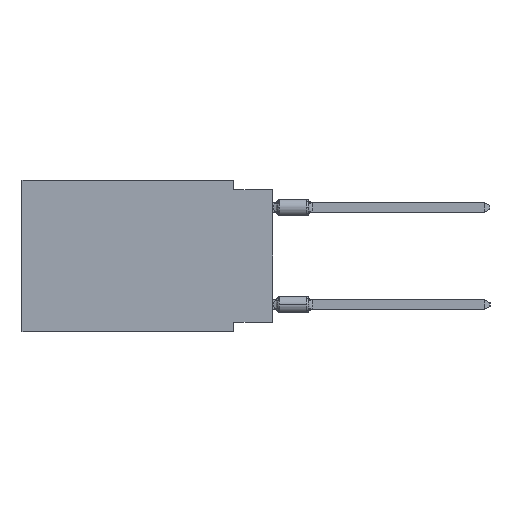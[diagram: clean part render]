
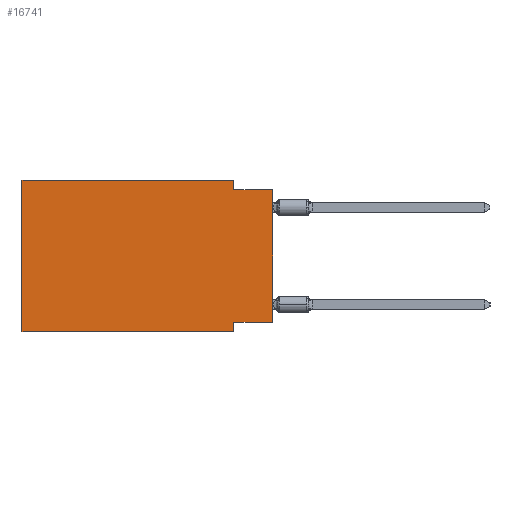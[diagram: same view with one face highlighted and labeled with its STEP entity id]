
A CAD part, left-side view. The second image highlights one B-rep face of the part: STEP entity #16741.
In plain terms, the highlighted planar face has unit normal (-1, 0, 0).
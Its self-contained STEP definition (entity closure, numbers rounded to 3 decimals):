
#205 = ORIENTED_EDGE ( 'NONE', *, *, #2849, .T. ) ;
#939 = EDGE_CURVE ( 'NONE', #19155, #3711, #29981, .T. ) ;
#1609 = CARTESIAN_POINT ( 'NONE',  ( 0., 0., -0.635 ) ) ;
#1792 = LINE ( 'NONE', #2024, #34343 ) ;
#2024 = CARTESIAN_POINT ( 'NONE',  ( 0., 2.54, 0. ) ) ;
#2849 = EDGE_CURVE ( 'NONE', #19155, #4385, #19594, .T. ) ;
#3100 = DIRECTION ( 'NONE',  ( 0., 0., -1. ) ) ;
#3331 = CARTESIAN_POINT ( 'NONE',  ( 0., 2.54, -9.906 ) ) ;
#3711 = VERTEX_POINT ( 'NONE', #45637 ) ;
#3762 = ORIENTED_EDGE ( 'NONE', *, *, #43737, .F. ) ;
#4385 = VERTEX_POINT ( 'NONE', #47497 ) ;
#5010 = LINE ( 'NONE', #1609, #28268 ) ;
#6751 = CARTESIAN_POINT ( 'NONE',  ( 0., 16.383, 0. ) ) ;
#7453 = DIRECTION ( 'NONE',  ( 0., 0., -1. ) ) ;
#8773 = EDGE_CURVE ( 'NONE', #41549, #30461, #1792, .T. ) ;
#8780 = DIRECTION ( 'NONE',  ( 0., -1., 0. ) ) ;
#9137 = VECTOR ( 'NONE', #18567, 1000. ) ;
#10598 = CARTESIAN_POINT ( 'NONE',  ( 0., 2.54, 0. ) ) ;
#13600 = VERTEX_POINT ( 'NONE', #17166 ) ;
#14380 = CARTESIAN_POINT ( 'NONE',  ( 0., 16.383, 0. ) ) ;
#14560 = VECTOR ( 'NONE', #41555, 1000. ) ;
#15902 = VECTOR ( 'NONE', #7453, 1000. ) ;
#15955 = CARTESIAN_POINT ( 'NONE',  ( 0., 0., 0. ) ) ;
#16059 = EDGE_CURVE ( 'NONE', #31178, #13600, #42051, .T. ) ;
#16741 = ADVANCED_FACE ( 'NONE', ( #35404 ), #47547, .F. ) ;
#17166 = CARTESIAN_POINT ( 'NONE',  ( 0., 2.54, -9.906 ) ) ;
#17244 = DIRECTION ( 'NONE',  ( 0., -1., 0. ) ) ;
#17719 = CARTESIAN_POINT ( 'NONE',  ( 0., 16.383, 0. ) ) ;
#17754 = EDGE_CURVE ( 'NONE', #30461, #4385, #5010, .T. ) ;
#18567 = DIRECTION ( 'NONE',  ( 0., 1., 0. ) ) ;
#19155 = VERTEX_POINT ( 'NONE', #35832 ) ;
#19594 = LINE ( 'NONE', #15955, #33290 ) ;
#20043 = DIRECTION ( 'NONE',  ( 0., -1., 0. ) ) ;
#21623 = ORIENTED_EDGE ( 'NONE', *, *, #939, .F. ) ;
#22936 = CARTESIAN_POINT ( 'NONE',  ( 0., 0., -9.271 ) ) ;
#22998 = DIRECTION ( 'NONE',  ( 0., 0., 1. ) ) ;
#23193 = CARTESIAN_POINT ( 'NONE',  ( 0., 2.54, -0.635 ) ) ;
#24993 = EDGE_CURVE ( 'NONE', #46889, #41549, #25009, .T. ) ;
#25009 = LINE ( 'NONE', #17719, #28607 ) ;
#26446 = ORIENTED_EDGE ( 'NONE', *, *, #8773, .F. ) ;
#28111 = EDGE_CURVE ( 'NONE', #3711, #13600, #44375, .T. ) ;
#28268 = VECTOR ( 'NONE', #20043, 1000. ) ;
#28607 = VECTOR ( 'NONE', #17244, 1000. ) ;
#28971 = AXIS2_PLACEMENT_3D ( 'NONE', #6751, #36377, #3100 ) ;
#29757 = CARTESIAN_POINT ( 'NONE',  ( 0., 16.383, -9.906 ) ) ;
#29981 = LINE ( 'NONE', #22936, #9137 ) ;
#30461 = VERTEX_POINT ( 'NONE', #23193 ) ;
#31178 = VERTEX_POINT ( 'NONE', #29757 ) ;
#33290 = VECTOR ( 'NONE', #22998, 1000. ) ;
#34025 = LINE ( 'NONE', #37918, #14560 ) ;
#34343 = VECTOR ( 'NONE', #38711, 1000. ) ;
#35395 = ORIENTED_EDGE ( 'NONE', *, *, #16059, .T. ) ;
#35404 = FACE_OUTER_BOUND ( 'NONE', #43707, .T. ) ;
#35832 = CARTESIAN_POINT ( 'NONE',  ( 0., 0., -9.271 ) ) ;
#36377 = DIRECTION ( 'NONE',  ( 1., 0., 0. ) ) ;
#36874 = ORIENTED_EDGE ( 'NONE', *, *, #17754, .F. ) ;
#37918 = CARTESIAN_POINT ( 'NONE',  ( 0., 16.383, 0. ) ) ;
#38711 = DIRECTION ( 'NONE',  ( 0., 0., -1. ) ) ;
#40564 = VECTOR ( 'NONE', #8780, 1000. ) ;
#41549 = VERTEX_POINT ( 'NONE', #10598 ) ;
#41555 = DIRECTION ( 'NONE',  ( 0., 0., 1. ) ) ;
#42051 = LINE ( 'NONE', #45452, #40564 ) ;
#43707 = EDGE_LOOP ( 'NONE', ( #205, #36874, #26446, #45635, #3762, #35395, #46642, #21623 ) ) ;
#43737 = EDGE_CURVE ( 'NONE', #31178, #46889, #34025, .T. ) ;
#44375 = LINE ( 'NONE', #3331, #15902 ) ;
#45452 = CARTESIAN_POINT ( 'NONE',  ( 0., 16.383, -9.906 ) ) ;
#45635 = ORIENTED_EDGE ( 'NONE', *, *, #24993, .F. ) ;
#45637 = CARTESIAN_POINT ( 'NONE',  ( 0., 2.54, -9.271 ) ) ;
#46642 = ORIENTED_EDGE ( 'NONE', *, *, #28111, .F. ) ;
#46889 = VERTEX_POINT ( 'NONE', #14380 ) ;
#47497 = CARTESIAN_POINT ( 'NONE',  ( 0., 0., -0.635 ) ) ;
#47547 = PLANE ( 'NONE',  #28971 ) ;
